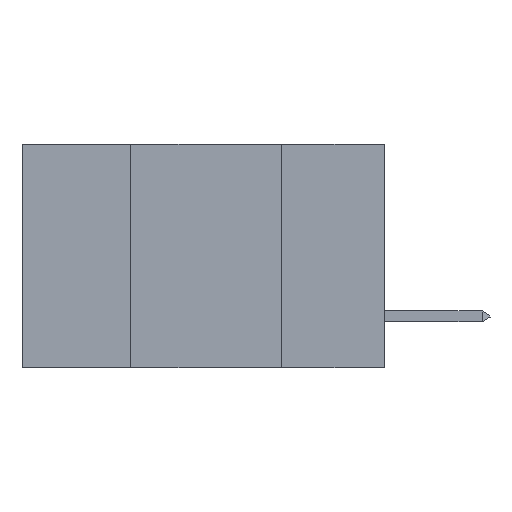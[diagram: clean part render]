
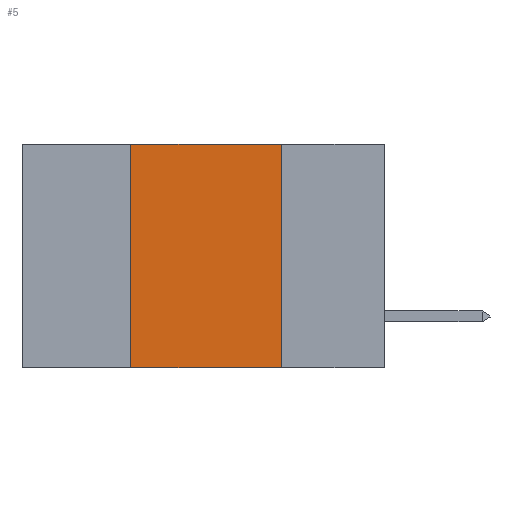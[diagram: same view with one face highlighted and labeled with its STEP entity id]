
A CAD part, left-side view. The second image highlights one B-rep face of the part: STEP entity #5.
In plain terms, the highlighted planar face has unit normal (-1, 0, 0).
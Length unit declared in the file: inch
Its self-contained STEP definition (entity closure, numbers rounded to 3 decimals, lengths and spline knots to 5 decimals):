
#5 = ADVANCED_FACE ( 'NONE', ( #15518 ), #23727, .F. ) ;
#197 = ORIENTED_EDGE ( 'NONE', *, *, #24850, .F. ) ;
#308 = DIRECTION ( 'NONE',  ( 0., -1., 0. ) ) ;
#1765 = ORIENTED_EDGE ( 'NONE', *, *, #32083, .F. ) ;
#1859 = EDGE_CURVE ( 'NONE', #21070, #21575, #32558, .T. ) ;
#1906 = CARTESIAN_POINT ( 'NONE',  ( 0., 0.17, 0. ) ) ;
#2497 = VECTOR ( 'NONE', #23272, 39.37008 ) ;
#3560 = DIRECTION ( 'NONE',  ( 0., 0., 1. ) ) ;
#5246 = VERTEX_POINT ( 'NONE', #6180 ) ;
#6180 = CARTESIAN_POINT ( 'NONE',  ( 0., 0.42, 0. ) ) ;
#8188 = AXIS2_PLACEMENT_3D ( 'NONE', #9913, #15076, #34550 ) ;
#9913 = CARTESIAN_POINT ( 'NONE',  ( 0., 0.6, 0. ) ) ;
#10143 = EDGE_LOOP ( 'NONE', ( #27868, #1765, #197, #20327 ) ) ;
#10970 = VECTOR ( 'NONE', #308, 39.37008 ) ;
#14745 = CARTESIAN_POINT ( 'NONE',  ( 0., 0.42, -0.37 ) ) ;
#14927 = VECTOR ( 'NONE', #3560, 39.37008 ) ;
#15076 = DIRECTION ( 'NONE',  ( 1., 0., 0. ) ) ;
#15518 = FACE_OUTER_BOUND ( 'NONE', #10143, .T. ) ;
#20327 = ORIENTED_EDGE ( 'NONE', *, *, #24560, .T. ) ;
#21070 = VERTEX_POINT ( 'NONE', #1906 ) ;
#21575 = VERTEX_POINT ( 'NONE', #23436 ) ;
#22988 = CARTESIAN_POINT ( 'NONE',  ( 0., 0.42, 0. ) ) ;
#23272 = DIRECTION ( 'NONE',  ( 0., -1., 0. ) ) ;
#23436 = CARTESIAN_POINT ( 'NONE',  ( 0., 0.17, -0.37 ) ) ;
#23727 = PLANE ( 'NONE',  #8188 ) ;
#24560 = EDGE_CURVE ( 'NONE', #25103, #21575, #26121, .T. ) ;
#24850 = EDGE_CURVE ( 'NONE', #25103, #5246, #34291, .T. ) ;
#25103 = VERTEX_POINT ( 'NONE', #14745 ) ;
#26121 = LINE ( 'NONE', #32062, #2497 ) ;
#26452 = LINE ( 'NONE', #30043, #10970 ) ;
#26945 = VECTOR ( 'NONE', #29688, 39.37008 ) ;
#27868 = ORIENTED_EDGE ( 'NONE', *, *, #1859, .F. ) ;
#29688 = DIRECTION ( 'NONE',  ( 0., 0., -1. ) ) ;
#30043 = CARTESIAN_POINT ( 'NONE',  ( 0., 0.6, 0. ) ) ;
#32062 = CARTESIAN_POINT ( 'NONE',  ( 0., 0.6, -0.37 ) ) ;
#32083 = EDGE_CURVE ( 'NONE', #5246, #21070, #26452, .T. ) ;
#32558 = LINE ( 'NONE', #35121, #26945 ) ;
#34291 = LINE ( 'NONE', #22988, #14927 ) ;
#34550 = DIRECTION ( 'NONE',  ( 0., 0., -1. ) ) ;
#35121 = CARTESIAN_POINT ( 'NONE',  ( 0., 0.17, 0. ) ) ;
